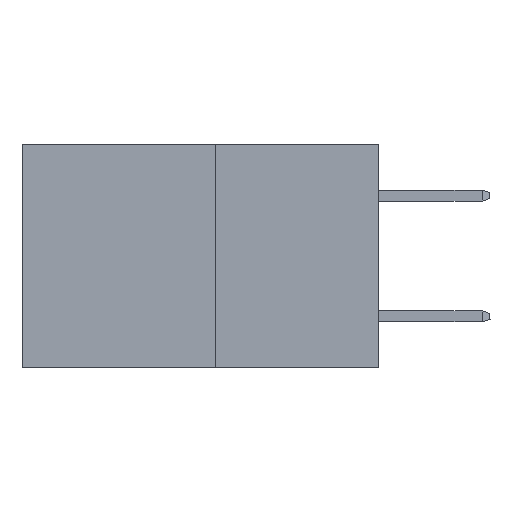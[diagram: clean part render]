
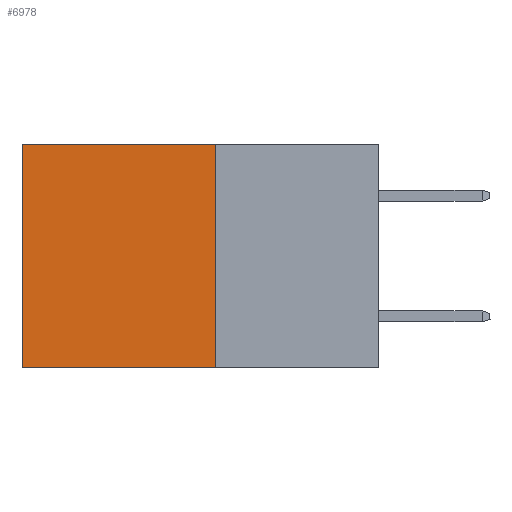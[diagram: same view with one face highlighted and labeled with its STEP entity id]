
A CAD part, left-side view. The second image highlights one B-rep face of the part: STEP entity #6978.
In plain terms, the highlighted planar face has unit normal (-1, 0, 0).
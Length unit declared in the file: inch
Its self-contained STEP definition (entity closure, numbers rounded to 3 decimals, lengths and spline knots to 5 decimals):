
#1283 = VECTOR ( 'NONE', #19376, 39.37008 ) ;
#1640 = CARTESIAN_POINT ( 'NONE',  ( 0.277, 0.27, 0. ) ) ;
#2707 = LINE ( 'NONE', #4927, #1283 ) ;
#3402 = CARTESIAN_POINT ( 'NONE',  ( 0.277, 0.59, -0.37 ) ) ;
#3898 = DIRECTION ( 'NONE',  ( 0., 0., -1. ) ) ;
#4927 = CARTESIAN_POINT ( 'NONE',  ( 0.277, 0.27, 0. ) ) ;
#5014 = ORIENTED_EDGE ( 'NONE', *, *, #26407, .F. ) ;
#6978 = ADVANCED_FACE ( 'NONE', ( #14021 ), #8833, .F. ) ;
#8595 = EDGE_CURVE ( 'NONE', #12742, #13978, #2707, .T. ) ;
#8687 = VECTOR ( 'NONE', #13709, 39.37008 ) ;
#8833 = PLANE ( 'NONE',  #18082 ) ;
#9321 = LINE ( 'NONE', #16295, #25704 ) ;
#10789 = VECTOR ( 'NONE', #11634, 39.37008 ) ;
#10915 = DIRECTION ( 'NONE',  ( 0., 0., -1. ) ) ;
#11634 = DIRECTION ( 'NONE',  ( 0., 1., 0. ) ) ;
#12631 = EDGE_CURVE ( 'NONE', #13978, #16278, #25094, .T. ) ;
#12742 = VERTEX_POINT ( 'NONE', #1640 ) ;
#12934 = CARTESIAN_POINT ( 'NONE',  ( 0.277, 0.27, -0.37 ) ) ;
#13709 = DIRECTION ( 'NONE',  ( 0., 0., -1. ) ) ;
#13978 = VERTEX_POINT ( 'NONE', #15905 ) ;
#14021 = FACE_OUTER_BOUND ( 'NONE', #15789, .T. ) ;
#14735 = ORIENTED_EDGE ( 'NONE', *, *, #12631, .T. ) ;
#14876 = ORIENTED_EDGE ( 'NONE', *, *, #16741, .F. ) ;
#15789 = EDGE_LOOP ( 'NONE', ( #14735, #5014, #14876, #23278 ) ) ;
#15905 = CARTESIAN_POINT ( 'NONE',  ( 0.277, 0.59, 0. ) ) ;
#16278 = VERTEX_POINT ( 'NONE', #25064 ) ;
#16295 = CARTESIAN_POINT ( 'NONE',  ( 0.277, 0.27, -0.37 ) ) ;
#16741 = EDGE_CURVE ( 'NONE', #12742, #26314, #9321, .T. ) ;
#17486 = CARTESIAN_POINT ( 'NONE',  ( 0.277, 0.27, -0.37 ) ) ;
#18082 = AXIS2_PLACEMENT_3D ( 'NONE', #12934, #23247, #10915 ) ;
#19376 = DIRECTION ( 'NONE',  ( 0., 1., 0. ) ) ;
#21767 = LINE ( 'NONE', #21892, #10789 ) ;
#21892 = CARTESIAN_POINT ( 'NONE',  ( 0.277, 0.27, -0.37 ) ) ;
#23247 = DIRECTION ( 'NONE',  ( 1., 0., 0. ) ) ;
#23278 = ORIENTED_EDGE ( 'NONE', *, *, #8595, .T. ) ;
#25064 = CARTESIAN_POINT ( 'NONE',  ( 0.277, 0.59, -0.37 ) ) ;
#25094 = LINE ( 'NONE', #3402, #8687 ) ;
#25704 = VECTOR ( 'NONE', #3898, 39.37008 ) ;
#26314 = VERTEX_POINT ( 'NONE', #17486 ) ;
#26407 = EDGE_CURVE ( 'NONE', #26314, #16278, #21767, .T. ) ;
